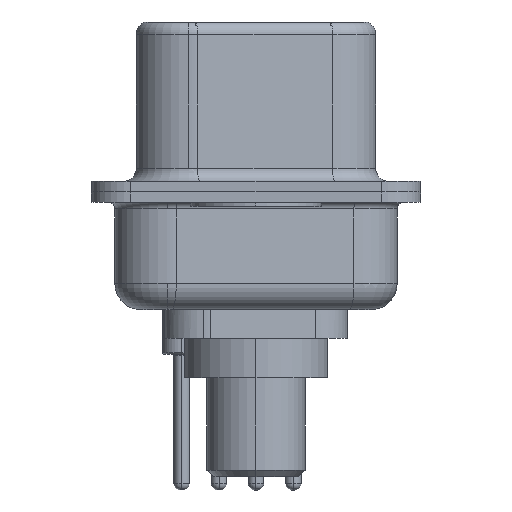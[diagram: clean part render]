
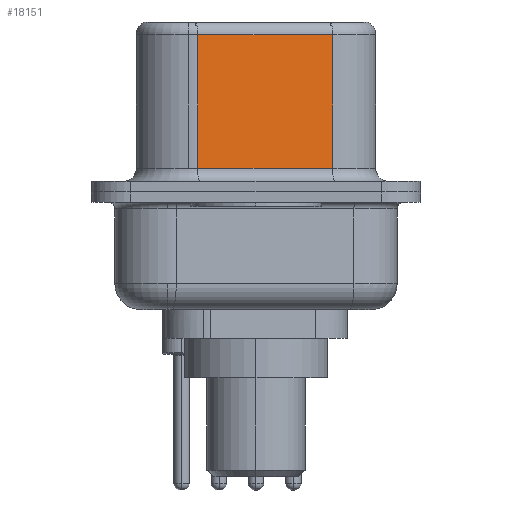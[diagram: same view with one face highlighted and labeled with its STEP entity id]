
A CAD part, left-side view. The second image highlights one B-rep face of the part: STEP entity #18151.
In plain terms, the highlighted planar face has unit normal (-0.985, -0.174, 0).
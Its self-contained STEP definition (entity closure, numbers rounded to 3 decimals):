
#109 = CARTESIAN_POINT ( 'NONE',  ( 3.67, 2.233, 6.52 ) ) ;
#112 = VERTEX_POINT ( 'NONE', #13041 ) ;
#829 = ORIENTED_EDGE ( 'NONE', *, *, #11243, .T. ) ;
#1425 = LINE ( 'NONE', #7125, #8536 ) ;
#1500 = EDGE_LOOP ( 'NONE', ( #16517, #8036, #12339, #829 ) ) ;
#2530 = CARTESIAN_POINT ( 'NONE',  ( 4.58, -2.927, 6.02 ) ) ;
#3856 = VECTOR ( 'NONE', #8703, 1000. ) ;
#4100 = FACE_OUTER_BOUND ( 'NONE', #1500, .T. ) ;
#5299 = CARTESIAN_POINT ( 'NONE',  ( 4.58, -2.927, 6.52 ) ) ;
#5717 = VERTEX_POINT ( 'NONE', #15402 ) ;
#6050 = CARTESIAN_POINT ( 'NONE',  ( 3.67, 2.233, 0.9 ) ) ;
#7125 = CARTESIAN_POINT ( 'NONE',  ( 4.58, -2.927, 6.52 ) ) ;
#8036 = ORIENTED_EDGE ( 'NONE', *, *, #10956, .T. ) ;
#8086 = LINE ( 'NONE', #15824, #3856 ) ;
#8116 = PLANE ( 'NONE',  #17000 ) ;
#8536 = VECTOR ( 'NONE', #9904, 1000. ) ;
#8703 = DIRECTION ( 'NONE',  ( 0.174, -0.985, 0. ) ) ;
#9349 = EDGE_CURVE ( 'NONE', #112, #14330, #14846, .T. ) ;
#9526 = DIRECTION ( 'NONE',  ( -0.174, 0.985, 0. ) ) ;
#9904 = DIRECTION ( 'NONE',  ( 0., 0., -1. ) ) ;
#10079 = LINE ( 'NONE', #13593, #16353 ) ;
#10956 = EDGE_CURVE ( 'NONE', #11103, #112, #10079, .T. ) ;
#11103 = VERTEX_POINT ( 'NONE', #2530 ) ;
#11187 = EDGE_CURVE ( 'NONE', #11103, #5717, #1425, .T. ) ;
#11243 = EDGE_CURVE ( 'NONE', #14330, #5717, #8086, .T. ) ;
#12339 = ORIENTED_EDGE ( 'NONE', *, *, #9349, .T. ) ;
#13041 = CARTESIAN_POINT ( 'NONE',  ( 3.67, 2.233, 6.02 ) ) ;
#13593 = CARTESIAN_POINT ( 'NONE',  ( 4.58, -2.927, 6.02 ) ) ;
#14330 = VERTEX_POINT ( 'NONE', #6050 ) ;
#14381 = VECTOR ( 'NONE', #17230, 1000. ) ;
#14846 = LINE ( 'NONE', #109, #14381 ) ;
#15402 = CARTESIAN_POINT ( 'NONE',  ( 4.58, -2.927, 0.9 ) ) ;
#15824 = CARTESIAN_POINT ( 'NONE',  ( 4.58, -2.927, 0.9 ) ) ;
#16353 = VECTOR ( 'NONE', #17842, 1000. ) ;
#16517 = ORIENTED_EDGE ( 'NONE', *, *, #11187, .F. ) ;
#17000 = AXIS2_PLACEMENT_3D ( 'NONE', #5299, #18071, #9526 ) ;
#17230 = DIRECTION ( 'NONE',  ( 0., 0., -1. ) ) ;
#17842 = DIRECTION ( 'NONE',  ( -0.174, 0.985, 0. ) ) ;
#18071 = DIRECTION ( 'NONE',  ( 0.985, 0.174, 0. ) ) ;
#18151 = ADVANCED_FACE ( 'NONE', ( #4100 ), #8116, .F. ) ;
